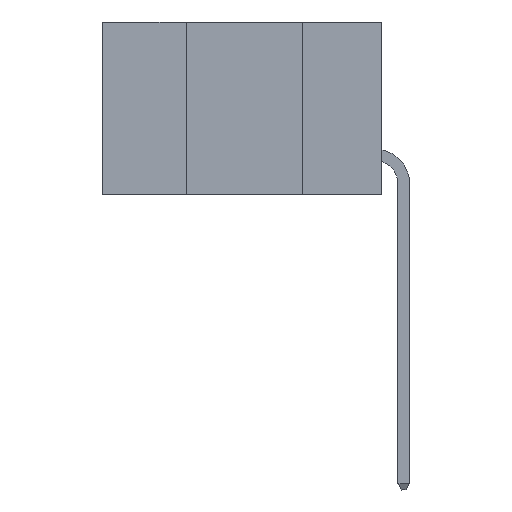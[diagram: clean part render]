
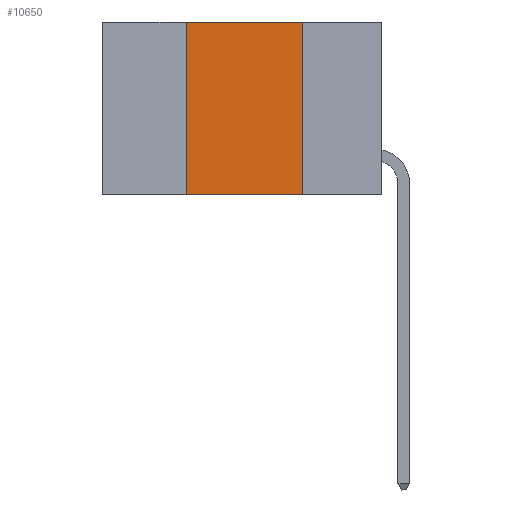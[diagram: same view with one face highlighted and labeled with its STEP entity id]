
A CAD part, left-side view. The second image highlights one B-rep face of the part: STEP entity #10650.
In plain terms, the highlighted planar face has unit normal (-1, 0, 0).
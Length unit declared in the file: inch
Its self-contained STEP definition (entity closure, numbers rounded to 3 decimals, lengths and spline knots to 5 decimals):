
#2489 = DIRECTION ( 'NONE',  ( 0., 0., -1. ) ) ;
#3635 = VERTEX_POINT ( 'NONE', #9777 ) ;
#4339 = EDGE_CURVE ( 'NONE', #12788, #3635, #14315, .T. ) ;
#4389 = VECTOR ( 'NONE', #2489, 39.37008 ) ;
#4513 = EDGE_CURVE ( 'NONE', #4915, #12788, #31567, .T. ) ;
#4841 = DIRECTION ( 'NONE',  ( 0., 0., 1. ) ) ;
#4915 = VERTEX_POINT ( 'NONE', #14678 ) ;
#5668 = CARTESIAN_POINT ( 'NONE',  ( 0., 0.6, 0. ) ) ;
#7389 = FACE_OUTER_BOUND ( 'NONE', #11163, .T. ) ;
#8394 = PLANE ( 'NONE',  #8896 ) ;
#8583 = CARTESIAN_POINT ( 'NONE',  ( 0., 0.17, -0.37 ) ) ;
#8896 = AXIS2_PLACEMENT_3D ( 'NONE', #5668, #21773, #27288 ) ;
#9219 = VECTOR ( 'NONE', #4841, 39.37008 ) ;
#9777 = CARTESIAN_POINT ( 'NONE',  ( 0., 0.17, 0. ) ) ;
#10650 = ADVANCED_FACE ( 'NONE', ( #7389 ), #8394, .F. ) ;
#11163 = EDGE_LOOP ( 'NONE', ( #23462, #33890, #20008, #27728 ) ) ;
#11611 = LINE ( 'NONE', #21274, #4389 ) ;
#12788 = VERTEX_POINT ( 'NONE', #19284 ) ;
#14315 = LINE ( 'NONE', #20615, #27816 ) ;
#14678 = CARTESIAN_POINT ( 'NONE',  ( 0., 0.42, -0.37 ) ) ;
#17243 = EDGE_CURVE ( 'NONE', #3635, #27652, #11611, .T. ) ;
#19284 = CARTESIAN_POINT ( 'NONE',  ( 0., 0.42, 0. ) ) ;
#20008 = ORIENTED_EDGE ( 'NONE', *, *, #4513, .F. ) ;
#20615 = CARTESIAN_POINT ( 'NONE',  ( 0., 0.6, 0. ) ) ;
#20658 = LINE ( 'NONE', #26052, #28635 ) ;
#21274 = CARTESIAN_POINT ( 'NONE',  ( 0., 0.17, 0. ) ) ;
#21773 = DIRECTION ( 'NONE',  ( 1., 0., 0. ) ) ;
#23335 = DIRECTION ( 'NONE',  ( 0., -1., 0. ) ) ;
#23462 = ORIENTED_EDGE ( 'NONE', *, *, #17243, .F. ) ;
#23926 = CARTESIAN_POINT ( 'NONE',  ( 0., 0.42, 0. ) ) ;
#26052 = CARTESIAN_POINT ( 'NONE',  ( 0., 0.6, -0.37 ) ) ;
#27288 = DIRECTION ( 'NONE',  ( 0., 0., -1. ) ) ;
#27652 = VERTEX_POINT ( 'NONE', #8583 ) ;
#27728 = ORIENTED_EDGE ( 'NONE', *, *, #30521, .T. ) ;
#27816 = VECTOR ( 'NONE', #23335, 39.37008 ) ;
#28635 = VECTOR ( 'NONE', #28728, 39.37008 ) ;
#28728 = DIRECTION ( 'NONE',  ( 0., -1., 0. ) ) ;
#30521 = EDGE_CURVE ( 'NONE', #4915, #27652, #20658, .T. ) ;
#31567 = LINE ( 'NONE', #23926, #9219 ) ;
#33890 = ORIENTED_EDGE ( 'NONE', *, *, #4339, .F. ) ;
